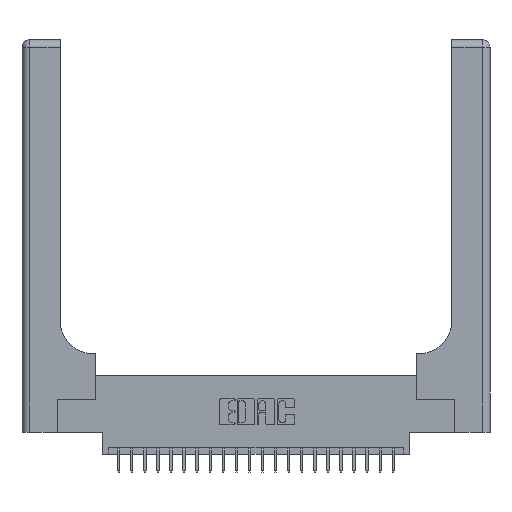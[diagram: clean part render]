
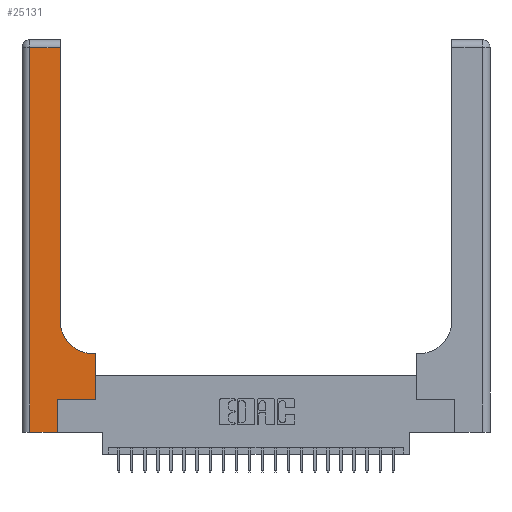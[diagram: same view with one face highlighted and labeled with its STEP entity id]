
A CAD part, top view. The second image highlights one B-rep face of the part: STEP entity #25131.
In plain terms, the highlighted planar face has unit normal (0, 0, 1).
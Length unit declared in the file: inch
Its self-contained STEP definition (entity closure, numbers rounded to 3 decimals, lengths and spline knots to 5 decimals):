
#667 = VECTOR ( 'NONE', #10368, 39.37008 ) ;
#886 = EDGE_CURVE ( 'NONE', #10582, #11267, #5797, .T. ) ;
#1871 = CARTESIAN_POINT ( 'NONE',  ( 0.2915, 0.85, 0.37 ) ) ;
#2158 = ORIENTED_EDGE ( 'NONE', *, *, #8696, .T. ) ;
#2229 = LINE ( 'NONE', #23808, #20793 ) ;
#2255 = LINE ( 'NONE', #13783, #19923 ) ;
#2526 = CARTESIAN_POINT ( 'NONE',  ( 0.5415, 0.6, 0.37 ) ) ;
#2943 = EDGE_CURVE ( 'NONE', #11267, #20988, #13898, .T. ) ;
#3148 = FACE_OUTER_BOUND ( 'NONE', #15727, .T. ) ;
#3277 = ORIENTED_EDGE ( 'NONE', *, *, #23278, .T. ) ;
#3279 = DIRECTION ( 'NONE',  ( -1., 0., 0. ) ) ;
#3309 = VERTEX_POINT ( 'NONE', #10265 ) ;
#3812 = VECTOR ( 'NONE', #19956, 39.37008 ) ;
#4314 = LINE ( 'NONE', #7888, #3812 ) ;
#4429 = CIRCLE ( 'NONE', #14231, 0.25 ) ;
#4587 = ORIENTED_EDGE ( 'NONE', *, *, #7096, .T. ) ;
#5237 = VECTOR ( 'NONE', #16320, 39.37008 ) ;
#5797 = LINE ( 'NONE', #13334, #15391 ) ;
#6274 = EDGE_CURVE ( 'NONE', #9227, #11221, #15273, .T. ) ;
#7096 = EDGE_CURVE ( 'NONE', #3309, #9227, #2255, .T. ) ;
#7387 = ORIENTED_EDGE ( 'NONE', *, *, #10601, .T. ) ;
#7888 = CARTESIAN_POINT ( 'NONE',  ( 0., 2.94, 0.37 ) ) ;
#8286 = CARTESIAN_POINT ( 'NONE',  ( 0.5585, 0.6, 0.37 ) ) ;
#8376 = VERTEX_POINT ( 'NONE', #2526 ) ;
#8696 = EDGE_CURVE ( 'NONE', #8376, #23646, #4429, .T. ) ;
#8948 = ORIENTED_EDGE ( 'NONE', *, *, #6274, .T. ) ;
#9040 = CARTESIAN_POINT ( 'NONE',  ( 0., 3., 0.37 ) ) ;
#9227 = VERTEX_POINT ( 'NONE', #18218 ) ;
#9295 = ORIENTED_EDGE ( 'NONE', *, *, #886, .T. ) ;
#9924 = CARTESIAN_POINT ( 'NONE',  ( 0.06, 2.94, 0.37 ) ) ;
#10265 = CARTESIAN_POINT ( 'NONE',  ( 0.269, 0.25, 0.37 ) ) ;
#10347 = CARTESIAN_POINT ( 'NONE',  ( 0.06, 0., 0.37 ) ) ;
#10368 = DIRECTION ( 'NONE',  ( 0., 1., 0. ) ) ;
#10582 = VERTEX_POINT ( 'NONE', #9924 ) ;
#10601 = EDGE_CURVE ( 'NONE', #20988, #3309, #2229, .T. ) ;
#10958 = PLANE ( 'NONE',  #18276 ) ;
#11221 = VERTEX_POINT ( 'NONE', #8286 ) ;
#11267 = VERTEX_POINT ( 'NONE', #10347 ) ;
#11423 = LINE ( 'NONE', #17439, #16167 ) ;
#11562 = DIRECTION ( 'NONE',  ( 0., -1., 0. ) ) ;
#13334 = CARTESIAN_POINT ( 'NONE',  ( 0.06, 3., 0.37 ) ) ;
#13783 = CARTESIAN_POINT ( 'NONE',  ( 0.269, 0.25, 0.37 ) ) ;
#13898 = LINE ( 'NONE', #21767, #5237 ) ;
#14231 = AXIS2_PLACEMENT_3D ( 'NONE', #17244, #15436, #23306 ) ;
#15273 = LINE ( 'NONE', #24778, #16126 ) ;
#15391 = VECTOR ( 'NONE', #11562, 39.37008 ) ;
#15436 = DIRECTION ( 'NONE',  ( 0., 0., -1. ) ) ;
#15638 = DIRECTION ( 'NONE',  ( -1., 0., 0. ) ) ;
#15727 = EDGE_LOOP ( 'NONE', ( #3277, #22003, #9295, #22885, #7387, #4587, #8948, #17298, #2158 ) ) ;
#16126 = VECTOR ( 'NONE', #19000, 39.37008 ) ;
#16167 = VECTOR ( 'NONE', #15638, 39.37008 ) ;
#16320 = DIRECTION ( 'NONE',  ( 1., 0., 0. ) ) ;
#17244 = CARTESIAN_POINT ( 'NONE',  ( 0.5415, 0.85, 0.37 ) ) ;
#17298 = ORIENTED_EDGE ( 'NONE', *, *, #22083, .T. ) ;
#17439 = CARTESIAN_POINT ( 'NONE',  ( 0.2915, 0.6, 0.37 ) ) ;
#17634 = CARTESIAN_POINT ( 'NONE',  ( 0.2915, 2.94, 0.37 ) ) ;
#18218 = CARTESIAN_POINT ( 'NONE',  ( 0.5585, 0.25, 0.37 ) ) ;
#18276 = AXIS2_PLACEMENT_3D ( 'NONE', #9040, #22783, #3279 ) ;
#18380 = EDGE_CURVE ( 'NONE', #20098, #10582, #4314, .T. ) ;
#19000 = DIRECTION ( 'NONE',  ( 0., 1., 0. ) ) ;
#19489 = CARTESIAN_POINT ( 'NONE',  ( 0.269, 0., 0.37 ) ) ;
#19858 = CARTESIAN_POINT ( 'NONE',  ( 0.2915, 3., 0.37 ) ) ;
#19923 = VECTOR ( 'NONE', #23576, 39.37008 ) ;
#19956 = DIRECTION ( 'NONE',  ( -1., 0., 0. ) ) ;
#20098 = VERTEX_POINT ( 'NONE', #17634 ) ;
#20793 = VECTOR ( 'NONE', #21875, 39.37008 ) ;
#20988 = VERTEX_POINT ( 'NONE', #19489 ) ;
#21767 = CARTESIAN_POINT ( 'NONE',  ( 0., 0., 0.37 ) ) ;
#21811 = LINE ( 'NONE', #19858, #667 ) ;
#21875 = DIRECTION ( 'NONE',  ( 0., 1., 0. ) ) ;
#22003 = ORIENTED_EDGE ( 'NONE', *, *, #18380, .T. ) ;
#22083 = EDGE_CURVE ( 'NONE', #11221, #8376, #11423, .T. ) ;
#22783 = DIRECTION ( 'NONE',  ( 0., 0., -1. ) ) ;
#22885 = ORIENTED_EDGE ( 'NONE', *, *, #2943, .T. ) ;
#23278 = EDGE_CURVE ( 'NONE', #23646, #20098, #21811, .T. ) ;
#23306 = DIRECTION ( 'NONE',  ( 1., 0., 0. ) ) ;
#23576 = DIRECTION ( 'NONE',  ( 1., 0., 0. ) ) ;
#23646 = VERTEX_POINT ( 'NONE', #1871 ) ;
#23808 = CARTESIAN_POINT ( 'NONE',  ( 0.269, 0., 0.37 ) ) ;
#24778 = CARTESIAN_POINT ( 'NONE',  ( 0.5585, 0.25, 0.37 ) ) ;
#25131 = ADVANCED_FACE ( 'NONE', ( #3148 ), #10958, .F. ) ;
